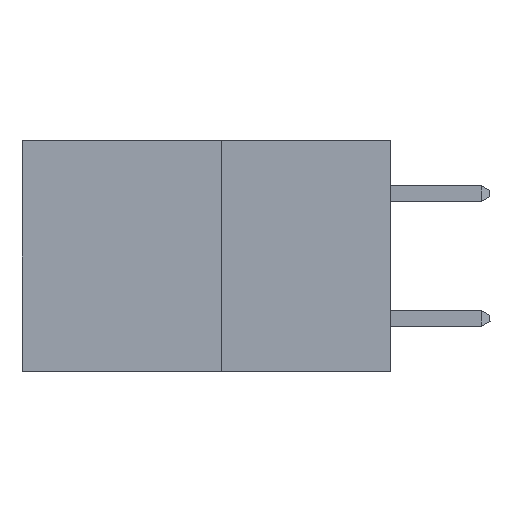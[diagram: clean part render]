
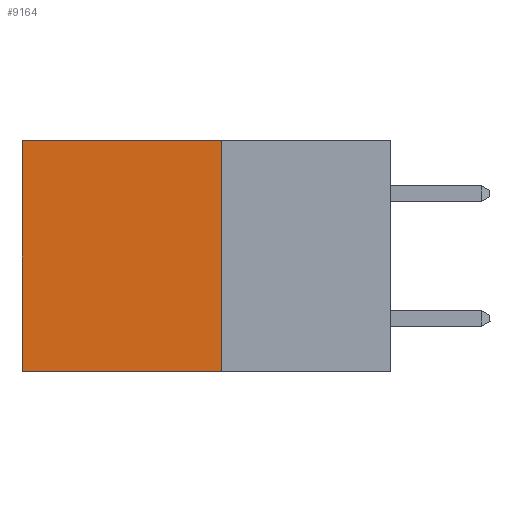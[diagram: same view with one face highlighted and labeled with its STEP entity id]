
A CAD part, left-side view. The second image highlights one B-rep face of the part: STEP entity #9164.
In plain terms, the highlighted planar face has unit normal (-1, 0, 0).
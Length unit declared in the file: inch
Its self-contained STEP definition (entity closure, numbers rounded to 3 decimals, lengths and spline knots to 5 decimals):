
#568 = VERTEX_POINT ( 'NONE', #8523 ) ;
#642 = EDGE_LOOP ( 'NONE', ( #15715, #10167, #1107, #1256 ) ) ;
#800 = VERTEX_POINT ( 'NONE', #21998 ) ;
#1092 = EDGE_CURVE ( 'NONE', #800, #11378, #6669, .T. ) ;
#1107 = ORIENTED_EDGE ( 'NONE', *, *, #1092, .F. ) ;
#1256 = ORIENTED_EDGE ( 'NONE', *, *, #19801, .T. ) ;
#1400 = DIRECTION ( 'NONE',  ( 1., 0., 0. ) ) ;
#1963 = VECTOR ( 'NONE', #5688, 39.37008 ) ;
#3619 = CARTESIAN_POINT ( 'NONE',  ( 0.277, 0.27, -0.37 ) ) ;
#3734 = DIRECTION ( 'NONE',  ( 0., 1., 0. ) ) ;
#4030 = CARTESIAN_POINT ( 'NONE',  ( 0.277, 0.59, 0. ) ) ;
#4530 = CARTESIAN_POINT ( 'NONE',  ( 0.277, 0.27, 0. ) ) ;
#5431 = LINE ( 'NONE', #9820, #18257 ) ;
#5688 = DIRECTION ( 'NONE',  ( 0., 0., -1. ) ) ;
#6669 = LINE ( 'NONE', #3619, #1963 ) ;
#6875 = EDGE_CURVE ( 'NONE', #14299, #568, #5431, .T. ) ;
#8054 = AXIS2_PLACEMENT_3D ( 'NONE', #8417, #1400, #13678 ) ;
#8417 = CARTESIAN_POINT ( 'NONE',  ( 0.277, 0.27, -0.37 ) ) ;
#8523 = CARTESIAN_POINT ( 'NONE',  ( 0.277, 0.59, -0.37 ) ) ;
#9164 = ADVANCED_FACE ( 'NONE', ( #19516 ), #11924, .F. ) ;
#9619 = DIRECTION ( 'NONE',  ( 0., 0., -1. ) ) ;
#9820 = CARTESIAN_POINT ( 'NONE',  ( 0.277, 0.59, -0.37 ) ) ;
#9988 = EDGE_CURVE ( 'NONE', #11378, #568, #11935, .T. ) ;
#10167 = ORIENTED_EDGE ( 'NONE', *, *, #9988, .F. ) ;
#10834 = VECTOR ( 'NONE', #18490, 39.37008 ) ;
#11377 = LINE ( 'NONE', #4530, #10834 ) ;
#11378 = VERTEX_POINT ( 'NONE', #16466 ) ;
#11924 = PLANE ( 'NONE',  #8054 ) ;
#11935 = LINE ( 'NONE', #15970, #21593 ) ;
#13678 = DIRECTION ( 'NONE',  ( 0., 0., -1. ) ) ;
#14299 = VERTEX_POINT ( 'NONE', #4030 ) ;
#15715 = ORIENTED_EDGE ( 'NONE', *, *, #6875, .T. ) ;
#15970 = CARTESIAN_POINT ( 'NONE',  ( 0.277, 0.27, -0.37 ) ) ;
#16466 = CARTESIAN_POINT ( 'NONE',  ( 0.277, 0.27, -0.37 ) ) ;
#18257 = VECTOR ( 'NONE', #9619, 39.37008 ) ;
#18490 = DIRECTION ( 'NONE',  ( 0., 1., 0. ) ) ;
#19516 = FACE_OUTER_BOUND ( 'NONE', #642, .T. ) ;
#19801 = EDGE_CURVE ( 'NONE', #800, #14299, #11377, .T. ) ;
#21593 = VECTOR ( 'NONE', #3734, 39.37008 ) ;
#21998 = CARTESIAN_POINT ( 'NONE',  ( 0.277, 0.27, 0. ) ) ;
